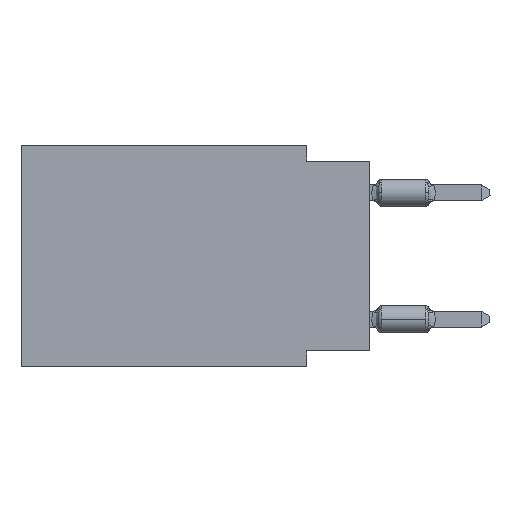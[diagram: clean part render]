
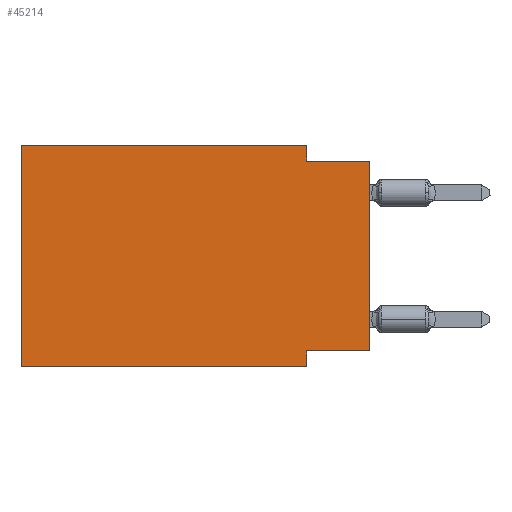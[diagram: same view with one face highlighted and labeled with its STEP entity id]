
A CAD part, left-side view. The second image highlights one B-rep face of the part: STEP entity #45214.
In plain terms, the highlighted planar face has unit normal (-1, 0, 0).
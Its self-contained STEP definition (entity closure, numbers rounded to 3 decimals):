
#275 = VERTEX_POINT ( 'NONE', #54719 ) ;
#1253 = VECTOR ( 'NONE', #31854, 1000. ) ;
#1636 = LINE ( 'NONE', #38733, #18212 ) ;
#2677 = LINE ( 'NONE', #20646, #15406 ) ;
#2750 = PLANE ( 'NONE',  #8651 ) ;
#2831 = ORIENTED_EDGE ( 'NONE', *, *, #54873, .T. ) ;
#5720 = EDGE_CURVE ( 'NONE', #6432, #45143, #52250, .T. ) ;
#6373 = EDGE_CURVE ( 'NONE', #28428, #26386, #1636, .T. ) ;
#6432 = VERTEX_POINT ( 'NONE', #34320 ) ;
#7690 = DIRECTION ( 'NONE',  ( 0., -1., 0. ) ) ;
#8651 = AXIS2_PLACEMENT_3D ( 'NONE', #11903, #30156, #20719 ) ;
#8753 = DIRECTION ( 'NONE',  ( 0., 0., -1. ) ) ;
#8994 = VECTOR ( 'NONE', #18274, 1000. ) ;
#9266 = ORIENTED_EDGE ( 'NONE', *, *, #54729, .F. ) ;
#9289 = LINE ( 'NONE', #55549, #33165 ) ;
#9964 = ORIENTED_EDGE ( 'NONE', *, *, #6373, .T. ) ;
#11385 = CARTESIAN_POINT ( 'NONE',  ( 0., 13.97, -8.89 ) ) ;
#11860 = CARTESIAN_POINT ( 'NONE',  ( 0., 13.97, 0. ) ) ;
#11903 = CARTESIAN_POINT ( 'NONE',  ( 0., 13.97, 0. ) ) ;
#14583 = DIRECTION ( 'NONE',  ( 0., 1., 0. ) ) ;
#15037 = LINE ( 'NONE', #45998, #44770 ) ;
#15406 = VECTOR ( 'NONE', #7690, 1000. ) ;
#15439 = CARTESIAN_POINT ( 'NONE',  ( 0., 2.54, 0. ) ) ;
#17438 = DIRECTION ( 'NONE',  ( 0., 0., -1. ) ) ;
#17762 = EDGE_CURVE ( 'NONE', #275, #26386, #2677, .T. ) ;
#18212 = VECTOR ( 'NONE', #24596, 1000. ) ;
#18245 = ORIENTED_EDGE ( 'NONE', *, *, #45880, .F. ) ;
#18274 = DIRECTION ( 'NONE',  ( 0., 0., 1. ) ) ;
#20271 = CARTESIAN_POINT ( 'NONE',  ( 0., 2.54, -8.89 ) ) ;
#20646 = CARTESIAN_POINT ( 'NONE',  ( 0., 0., -0.635 ) ) ;
#20719 = DIRECTION ( 'NONE',  ( 0., 0., -1. ) ) ;
#22874 = LINE ( 'NONE', #50013, #56880 ) ;
#23553 = LINE ( 'NONE', #45980, #8994 ) ;
#24596 = DIRECTION ( 'NONE',  ( 0., 0., 1. ) ) ;
#26386 = VERTEX_POINT ( 'NONE', #34361 ) ;
#27048 = ORIENTED_EDGE ( 'NONE', *, *, #41229, .F. ) ;
#28234 = EDGE_CURVE ( 'NONE', #28428, #36024, #9289, .T. ) ;
#28428 = VERTEX_POINT ( 'NONE', #33975 ) ;
#30156 = DIRECTION ( 'NONE',  ( 1., 0., 0. ) ) ;
#31854 = DIRECTION ( 'NONE',  ( 0., -1., 0. ) ) ;
#32669 = ORIENTED_EDGE ( 'NONE', *, *, #28234, .F. ) ;
#33165 = VECTOR ( 'NONE', #14583, 1000. ) ;
#33975 = CARTESIAN_POINT ( 'NONE',  ( 0., 0., -8.255 ) ) ;
#34320 = CARTESIAN_POINT ( 'NONE',  ( 0., 13.97, 0. ) ) ;
#34361 = CARTESIAN_POINT ( 'NONE',  ( 0., 0., -0.635 ) ) ;
#34953 = EDGE_LOOP ( 'NONE', ( #9964, #57564, #27048, #57219, #18245, #2831, #9266, #32669 ) ) ;
#35294 = VECTOR ( 'NONE', #17438, 1000. ) ;
#36024 = VERTEX_POINT ( 'NONE', #57942 ) ;
#38733 = CARTESIAN_POINT ( 'NONE',  ( 0., 0., 0. ) ) ;
#41229 = EDGE_CURVE ( 'NONE', #45143, #275, #22874, .T. ) ;
#42423 = DIRECTION ( 'NONE',  ( 0., -1., 0. ) ) ;
#42847 = FACE_OUTER_BOUND ( 'NONE', #34953, .T. ) ;
#43472 = VERTEX_POINT ( 'NONE', #20271 ) ;
#44770 = VECTOR ( 'NONE', #42423, 1000. ) ;
#45143 = VERTEX_POINT ( 'NONE', #15439 ) ;
#45214 = ADVANCED_FACE ( 'NONE', ( #42847 ), #2750, .F. ) ;
#45880 = EDGE_CURVE ( 'NONE', #51127, #6432, #23553, .T. ) ;
#45980 = CARTESIAN_POINT ( 'NONE',  ( 0., 13.97, 0. ) ) ;
#45998 = CARTESIAN_POINT ( 'NONE',  ( 0., 13.97, -8.89 ) ) ;
#50013 = CARTESIAN_POINT ( 'NONE',  ( 0., 2.54, 0. ) ) ;
#51127 = VERTEX_POINT ( 'NONE', #11385 ) ;
#52250 = LINE ( 'NONE', #11860, #1253 ) ;
#54719 = CARTESIAN_POINT ( 'NONE',  ( 0., 2.54, -0.635 ) ) ;
#54729 = EDGE_CURVE ( 'NONE', #36024, #43472, #57842, .T. ) ;
#54873 = EDGE_CURVE ( 'NONE', #51127, #43472, #15037, .T. ) ;
#55549 = CARTESIAN_POINT ( 'NONE',  ( 0., 0., -8.255 ) ) ;
#56880 = VECTOR ( 'NONE', #8753, 1000. ) ;
#57219 = ORIENTED_EDGE ( 'NONE', *, *, #5720, .F. ) ;
#57564 = ORIENTED_EDGE ( 'NONE', *, *, #17762, .F. ) ;
#57842 = LINE ( 'NONE', #58140, #35294 ) ;
#57942 = CARTESIAN_POINT ( 'NONE',  ( 0., 2.54, -8.255 ) ) ;
#58140 = CARTESIAN_POINT ( 'NONE',  ( 0., 2.54, -8.89 ) ) ;
